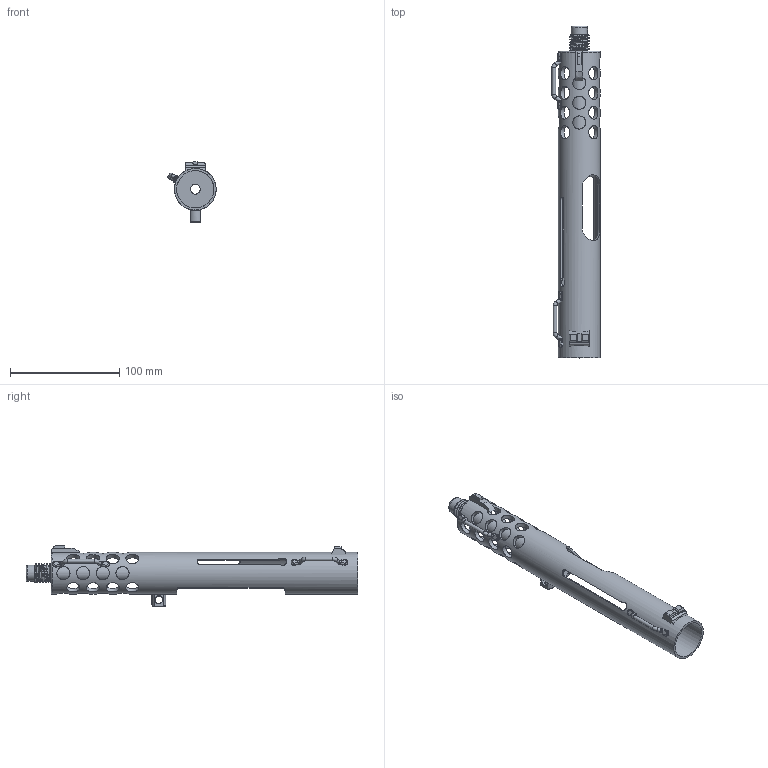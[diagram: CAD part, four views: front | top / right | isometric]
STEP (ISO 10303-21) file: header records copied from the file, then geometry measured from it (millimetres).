
FILE_DESCRIPTION(/* description */ (''),/* implementation_level */ '2;1');
FILE_NAME(/* name */ 'KG99 v1.step',/* time_stamp */ '2025-06-02T14:40:47-07:00',/* author */ (''),/* organization */ (''),/* preprocessor_version */ 'ST-DEVELOPER v20.1',/* originating_system */ 'Autodesk Translation Framework v14.10.0.0',/* authorisation */ '');
FILE_SCHEMA (('AUTOMOTIVE_DESIGN { 1 0 10303 214 3 1 1 }'));
Length unit declared in the file: millimetre
Products named in the file (1): KG99 v1 (1)
Bounding box: 44.14 x 303.5 x 55.5 mm (x, y, z)
Volume: 75119.8 mm3; surface area: 64866.4 mm2
Topology: 3 solids, 3 shells, 208 faces, 610 edges, 397 vertices
Faces by surface type: cylinder 99, plane 54, bspline 41, torus 10, cone 4
Full cylindrical faces by diameter (mm): 3.5 x6, 5 x2, 7 x1, 8 x1, 9 x1, 12 x31, 14.938 x6, 15 x2, 17.791 x6, 30.1 x1, 34.1 x1, 38.1 x1
Entity records: 12306 total; most frequent: CARTESIAN_POINT 7118, ORIENTED_EDGE 1204, DIRECTION 844, EDGE_CURVE 602, VERTEX_POINT 397, AXIS2_PLACEMENT_3D 325, EDGE_LOOP 279, B_SPLINE_CURVE_WITH_KNOTS 247
